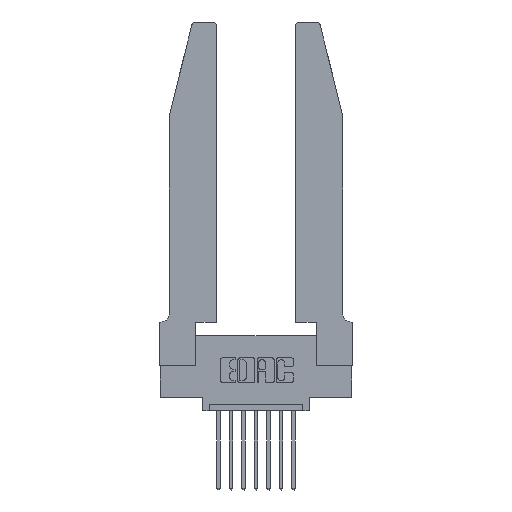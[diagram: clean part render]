
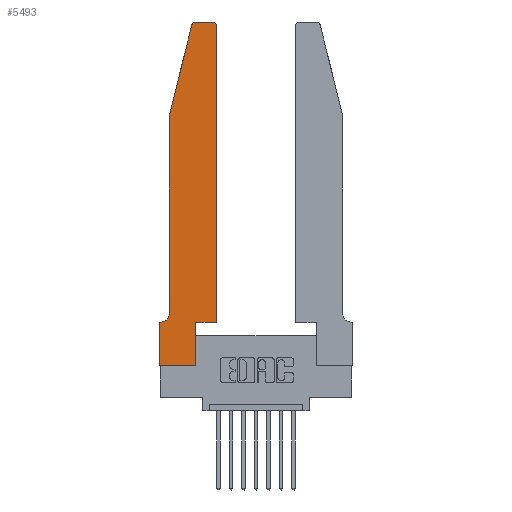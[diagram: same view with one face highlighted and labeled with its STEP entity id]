
A CAD part, top view. The second image highlights one B-rep face of the part: STEP entity #5493.
In plain terms, the highlighted planar face has unit normal (0, 0, 1).
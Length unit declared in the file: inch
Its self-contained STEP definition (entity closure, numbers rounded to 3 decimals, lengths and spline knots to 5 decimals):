
#136 = ORIENTED_EDGE ( 'NONE', *, *, #360, .T. ) ;
#318 = LINE ( 'NONE', #3394, #9083 ) ;
#329 = EDGE_CURVE ( 'NONE', #5782, #6876, #7739, .T. ) ;
#360 = EDGE_CURVE ( 'NONE', #1572, #7279, #3448, .T. ) ;
#458 = VERTEX_POINT ( 'NONE', #10608 ) ;
#833 = VERTEX_POINT ( 'NONE', #14826 ) ;
#902 = ORIENTED_EDGE ( 'NONE', *, *, #10803, .T. ) ;
#926 = DIRECTION ( 'NONE',  ( -1., 0., 0. ) ) ;
#1209 = EDGE_CURVE ( 'NONE', #458, #6954, #8407, .T. ) ;
#1297 = DIRECTION ( 'NONE',  ( 1., 0., 0. ) ) ;
#1332 = CARTESIAN_POINT ( 'NONE',  ( 0.4505, 0.35, 0.37 ) ) ;
#1351 = CIRCLE ( 'NONE', #5212, 0.03 ) ;
#1572 = VERTEX_POINT ( 'NONE', #11578 ) ;
#2154 = CARTESIAN_POINT ( 'NONE',  ( 0.0055, 0.42, 0.37 ) ) ;
#2208 = EDGE_LOOP ( 'NONE', ( #3290, #136, #7696, #12345, #902, #7678, #2251, #11253, #2506, #6612, #5638, #13768 ) ) ;
#2251 = ORIENTED_EDGE ( 'NONE', *, *, #11792, .T. ) ;
#2353 = DIRECTION ( 'NONE',  ( -1., 0., 0. ) ) ;
#2481 = AXIS2_PLACEMENT_3D ( 'NONE', #2154, #4498, #2353 ) ;
#2506 = ORIENTED_EDGE ( 'NONE', *, *, #329, .T. ) ;
#2668 = VECTOR ( 'NONE', #10205, 39.37008 ) ;
#2683 = VERTEX_POINT ( 'NONE', #11857 ) ;
#3125 = LINE ( 'NONE', #9198, #13686 ) ;
#3264 = LINE ( 'NONE', #3637, #10068 ) ;
#3290 = ORIENTED_EDGE ( 'NONE', *, *, #3411, .T. ) ;
#3394 = CARTESIAN_POINT ( 'NONE',  ( 0.0755, 0.35, 0.37 ) ) ;
#3407 = DIRECTION ( 'NONE',  ( 0., 0., 1. ) ) ;
#3411 = EDGE_CURVE ( 'NONE', #833, #1572, #8891, .T. ) ;
#3432 = EDGE_CURVE ( 'NONE', #8502, #833, #1351, .T. ) ;
#3448 = CIRCLE ( 'NONE', #7562, 0.03 ) ;
#3637 = CARTESIAN_POINT ( 'NONE',  ( 0., 0., 0.37 ) ) ;
#4177 = LINE ( 'NONE', #6411, #10970 ) ;
#4341 = CARTESIAN_POINT ( 'NONE',  ( 0., 0.35, 0.37 ) ) ;
#4378 = FACE_OUTER_BOUND ( 'NONE', #2208, .T. ) ;
#4446 = CARTESIAN_POINT ( 'NONE',  ( 0.2865, 0., 0.37 ) ) ;
#4498 = DIRECTION ( 'NONE',  ( 0., 0., -1. ) ) ;
#4559 = CARTESIAN_POINT ( 'NONE',  ( 0.0755, 2., 0.37 ) ) ;
#4880 = DIRECTION ( 'NONE',  ( 0., -1., 0. ) ) ;
#4911 = DIRECTION ( 'NONE',  ( 0., 0., 1. ) ) ;
#4940 = CARTESIAN_POINT ( 'NONE',  ( 0., 0., 0.37 ) ) ;
#5212 = AXIS2_PLACEMENT_3D ( 'NONE', #10253, #3407, #11433 ) ;
#5493 = ADVANCED_FACE ( 'NONE', ( #4378 ), #8859, .T. ) ;
#5638 = ORIENTED_EDGE ( 'NONE', *, *, #10525, .T. ) ;
#5782 = VERTEX_POINT ( 'NONE', #4446 ) ;
#5970 = DIRECTION ( 'NONE',  ( 0., 1., 0. ) ) ;
#6411 = CARTESIAN_POINT ( 'NONE',  ( 0.4505, 0.35, 0.37 ) ) ;
#6612 = ORIENTED_EDGE ( 'NONE', *, *, #8579, .T. ) ;
#6876 = VERTEX_POINT ( 'NONE', #8682 ) ;
#6954 = VERTEX_POINT ( 'NONE', #8548 ) ;
#7171 = CARTESIAN_POINT ( 'NONE',  ( 0.284, 2.72, 0.37 ) ) ;
#7187 = VECTOR ( 'NONE', #4880, 39.37008 ) ;
#7279 = VERTEX_POINT ( 'NONE', #12942 ) ;
#7562 = AXIS2_PLACEMENT_3D ( 'NONE', #7171, #4911, #11902 ) ;
#7678 = ORIENTED_EDGE ( 'NONE', *, *, #13541, .T. ) ;
#7696 = ORIENTED_EDGE ( 'NONE', *, *, #8126, .T. ) ;
#7733 = CIRCLE ( 'NONE', #2481, 0.07 ) ;
#7739 = LINE ( 'NONE', #12807, #13511 ) ;
#7990 = DIRECTION ( 'NONE',  ( -1., 0., 0. ) ) ;
#8126 = EDGE_CURVE ( 'NONE', #7279, #458, #3125, .T. ) ;
#8407 = LINE ( 'NONE', #4559, #2668 ) ;
#8502 = VERTEX_POINT ( 'NONE', #13865 ) ;
#8548 = CARTESIAN_POINT ( 'NONE',  ( 0.0755, 0.42, 0.37 ) ) ;
#8579 = EDGE_CURVE ( 'NONE', #6876, #2683, #14448, .T. ) ;
#8682 = CARTESIAN_POINT ( 'NONE',  ( 0.2865, 0.35, 0.37 ) ) ;
#8859 = PLANE ( 'NONE',  #11192 ) ;
#8891 = LINE ( 'NONE', #10156, #12330 ) ;
#8958 = DIRECTION ( 'NONE',  ( 0., 0., 1. ) ) ;
#9083 = VECTOR ( 'NONE', #926, 39.37008 ) ;
#9198 = CARTESIAN_POINT ( 'NONE',  ( 0.0755, 2., 0.37 ) ) ;
#9250 = DIRECTION ( 'NONE',  ( -0.239, -0.971, 0. ) ) ;
#9488 = VERTEX_POINT ( 'NONE', #4341 ) ;
#9781 = VERTEX_POINT ( 'NONE', #12861 ) ;
#10068 = VECTOR ( 'NONE', #11664, 39.37008 ) ;
#10156 = CARTESIAN_POINT ( 'NONE',  ( 0.2605, 2.75, 0.37 ) ) ;
#10205 = DIRECTION ( 'NONE',  ( 0., -1., 0. ) ) ;
#10215 = DIRECTION ( 'NONE',  ( 1., 0., 0. ) ) ;
#10253 = CARTESIAN_POINT ( 'NONE',  ( 0.4205, 2.72, 0.37 ) ) ;
#10525 = EDGE_CURVE ( 'NONE', #2683, #8502, #4177, .T. ) ;
#10608 = CARTESIAN_POINT ( 'NONE',  ( 0.0755, 2., 0.37 ) ) ;
#10803 = EDGE_CURVE ( 'NONE', #6954, #9781, #7733, .T. ) ;
#10918 = EDGE_CURVE ( 'NONE', #11045, #5782, #3264, .T. ) ;
#10944 = DIRECTION ( 'NONE',  ( 0., 1., 0. ) ) ;
#10970 = VECTOR ( 'NONE', #10944, 39.37008 ) ;
#11045 = VERTEX_POINT ( 'NONE', #12015 ) ;
#11192 = AXIS2_PLACEMENT_3D ( 'NONE', #12440, #8958, #10215 ) ;
#11253 = ORIENTED_EDGE ( 'NONE', *, *, #10918, .T. ) ;
#11433 = DIRECTION ( 'NONE',  ( 1., 0., 0. ) ) ;
#11578 = CARTESIAN_POINT ( 'NONE',  ( 0.284, 2.75, 0.37 ) ) ;
#11664 = DIRECTION ( 'NONE',  ( 1., 0., 0. ) ) ;
#11792 = EDGE_CURVE ( 'NONE', #9488, #11045, #14565, .T. ) ;
#11857 = CARTESIAN_POINT ( 'NONE',  ( 0.4505, 0.35, 0.37 ) ) ;
#11902 = DIRECTION ( 'NONE',  ( 1., 0., 0. ) ) ;
#12015 = CARTESIAN_POINT ( 'NONE',  ( 0., 0., 0.37 ) ) ;
#12330 = VECTOR ( 'NONE', #7990, 39.37008 ) ;
#12345 = ORIENTED_EDGE ( 'NONE', *, *, #1209, .T. ) ;
#12440 = CARTESIAN_POINT ( 'NONE',  ( 0., 0.35, 0.37 ) ) ;
#12807 = CARTESIAN_POINT ( 'NONE',  ( 0.2865, 0.35, 0.37 ) ) ;
#12861 = CARTESIAN_POINT ( 'NONE',  ( 0.0055, 0.35, 0.37 ) ) ;
#12942 = CARTESIAN_POINT ( 'NONE',  ( 0.25487, 2.72718, 0.37 ) ) ;
#13511 = VECTOR ( 'NONE', #5970, 39.37008 ) ;
#13541 = EDGE_CURVE ( 'NONE', #9781, #9488, #318, .T. ) ;
#13686 = VECTOR ( 'NONE', #9250, 39.37008 ) ;
#13768 = ORIENTED_EDGE ( 'NONE', *, *, #3432, .T. ) ;
#13865 = CARTESIAN_POINT ( 'NONE',  ( 0.4505, 2.72, 0.37 ) ) ;
#14448 = LINE ( 'NONE', #1332, #14643 ) ;
#14565 = LINE ( 'NONE', #4940, #7187 ) ;
#14643 = VECTOR ( 'NONE', #1297, 39.37008 ) ;
#14826 = CARTESIAN_POINT ( 'NONE',  ( 0.4205, 2.75, 0.37 ) ) ;
